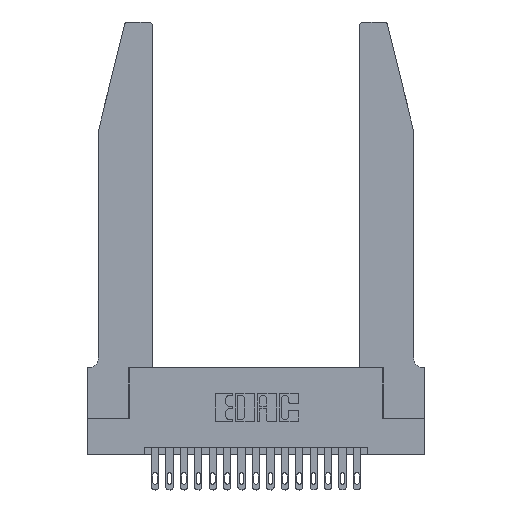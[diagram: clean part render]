
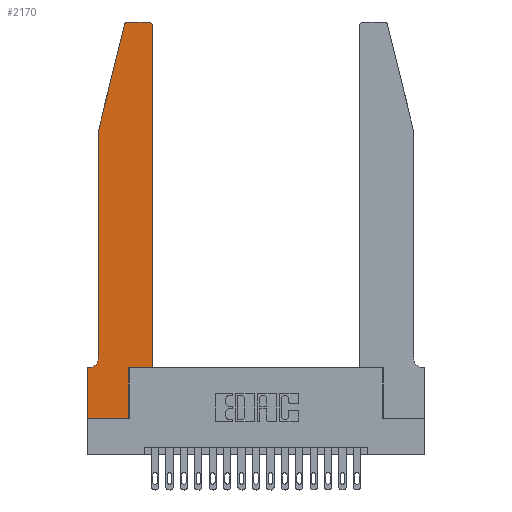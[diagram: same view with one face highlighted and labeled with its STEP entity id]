
A CAD part, top view. The second image highlights one B-rep face of the part: STEP entity #2170.
In plain terms, the highlighted planar face has unit normal (0, 0, 1).
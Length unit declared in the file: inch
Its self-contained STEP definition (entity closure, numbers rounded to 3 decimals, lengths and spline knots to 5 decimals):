
#248 = EDGE_CURVE ( 'NONE', #19533, #18526, #6119, .T. ) ;
#366 = DIRECTION ( 'NONE',  ( 1., 0., 0. ) ) ;
#376 = VERTEX_POINT ( 'NONE', #8955 ) ;
#439 = CARTESIAN_POINT ( 'NONE',  ( 0.0755, 0.35, 0.37 ) ) ;
#495 = VERTEX_POINT ( 'NONE', #17113 ) ;
#502 = EDGE_CURVE ( 'NONE', #8190, #19533, #6596, .T. ) ;
#740 = CARTESIAN_POINT ( 'NONE',  ( 0.2865, 0.35, 0.37 ) ) ;
#761 = ORIENTED_EDGE ( 'NONE', *, *, #19581, .T. ) ;
#892 = DIRECTION ( 'NONE',  ( -1., 0., 0. ) ) ;
#1048 = ORIENTED_EDGE ( 'NONE', *, *, #15730, .T. ) ;
#1582 = CARTESIAN_POINT ( 'NONE',  ( 0.0755, 0.42, 0.37 ) ) ;
#1654 = DIRECTION ( 'NONE',  ( 0., -1., 0. ) ) ;
#1697 = CARTESIAN_POINT ( 'NONE',  ( 0.4505, 0.35, 0.37 ) ) ;
#2170 = ADVANCED_FACE ( 'NONE', ( #5588 ), #3461, .T. ) ;
#3083 = EDGE_CURVE ( 'NONE', #18575, #8630, #14760, .T. ) ;
#3408 = AXIS2_PLACEMENT_3D ( 'NONE', #4958, #6515, #366 ) ;
#3455 = CARTESIAN_POINT ( 'NONE',  ( 0.4205, 2.75, 0.37 ) ) ;
#3461 = PLANE ( 'NONE',  #3408 ) ;
#3568 = CIRCLE ( 'NONE', #14250, 0.03 ) ;
#3593 = VERTEX_POINT ( 'NONE', #8522 ) ;
#3665 = LINE ( 'NONE', #19968, #15563 ) ;
#3952 = DIRECTION ( 'NONE',  ( 0., 0., 1. ) ) ;
#3953 = EDGE_CURVE ( 'NONE', #9859, #495, #4780, .T. ) ;
#4123 = EDGE_CURVE ( 'NONE', #14168, #9859, #5027, .T. ) ;
#4678 = CARTESIAN_POINT ( 'NONE',  ( 0., 0., 0.37 ) ) ;
#4702 = ORIENTED_EDGE ( 'NONE', *, *, #15828, .T. ) ;
#4780 = CIRCLE ( 'NONE', #11219, 0.07 ) ;
#4878 = CARTESIAN_POINT ( 'NONE',  ( 0.0755, 2., 0.37 ) ) ;
#4958 = CARTESIAN_POINT ( 'NONE',  ( 0., 0.35, 0.37 ) ) ;
#5027 = LINE ( 'NONE', #18552, #18361 ) ;
#5333 = EDGE_CURVE ( 'NONE', #3593, #18575, #12980, .T. ) ;
#5356 = ORIENTED_EDGE ( 'NONE', *, *, #248, .T. ) ;
#5588 = FACE_OUTER_BOUND ( 'NONE', #6091, .T. ) ;
#5661 = ORIENTED_EDGE ( 'NONE', *, *, #502, .T. ) ;
#5829 = LINE ( 'NONE', #8530, #14571 ) ;
#6091 = EDGE_LOOP ( 'NONE', ( #9227, #16138, #1048, #8426, #10344, #761, #7864, #5661, #5356, #4702, #13267, #17937 ) ) ;
#6119 = LINE ( 'NONE', #8564, #18029 ) ;
#6168 = VERTEX_POINT ( 'NONE', #17210 ) ;
#6281 = CARTESIAN_POINT ( 'NONE',  ( 0., 0., 0.37 ) ) ;
#6424 = DIRECTION ( 'NONE',  ( 0., 0., 1. ) ) ;
#6515 = DIRECTION ( 'NONE',  ( 0., 0., 1. ) ) ;
#6596 = LINE ( 'NONE', #17051, #9740 ) ;
#6760 = DIRECTION ( 'NONE',  ( 0., 0., -1. ) ) ;
#7532 = VECTOR ( 'NONE', #7723, 39.37008 ) ;
#7723 = DIRECTION ( 'NONE',  ( 1., 0., 0. ) ) ;
#7864 = ORIENTED_EDGE ( 'NONE', *, *, #14664, .T. ) ;
#8190 = VERTEX_POINT ( 'NONE', #4678 ) ;
#8325 = DIRECTION ( 'NONE',  ( -1., 0., 0. ) ) ;
#8426 = ORIENTED_EDGE ( 'NONE', *, *, #4123, .T. ) ;
#8522 = CARTESIAN_POINT ( 'NONE',  ( 0.4505, 0.35, 0.37 ) ) ;
#8530 = CARTESIAN_POINT ( 'NONE',  ( 0.2605, 2.75, 0.37 ) ) ;
#8564 = CARTESIAN_POINT ( 'NONE',  ( 0.2865, 0.35, 0.37 ) ) ;
#8630 = VERTEX_POINT ( 'NONE', #3455 ) ;
#8710 = DIRECTION ( 'NONE',  ( -1., 0., 0. ) ) ;
#8943 = DIRECTION ( 'NONE',  ( -0.239, -0.971, 0. ) ) ;
#8955 = CARTESIAN_POINT ( 'NONE',  ( 0.284, 2.75, 0.37 ) ) ;
#9227 = ORIENTED_EDGE ( 'NONE', *, *, #16183, .T. ) ;
#9392 = CARTESIAN_POINT ( 'NONE',  ( 0.4505, 0.35, 0.37 ) ) ;
#9740 = VECTOR ( 'NONE', #18667, 39.37008 ) ;
#9859 = VERTEX_POINT ( 'NONE', #1582 ) ;
#10344 = ORIENTED_EDGE ( 'NONE', *, *, #3953, .T. ) ;
#10961 = DIRECTION ( 'NONE',  ( 0., 1., 0. ) ) ;
#11219 = AXIS2_PLACEMENT_3D ( 'NONE', #14438, #6760, #8325 ) ;
#11280 = VECTOR ( 'NONE', #10961, 39.37008 ) ;
#11695 = CARTESIAN_POINT ( 'NONE',  ( 0.4505, 2.72, 0.37 ) ) ;
#11909 = LINE ( 'NONE', #6281, #18731 ) ;
#12718 = LINE ( 'NONE', #439, #13212 ) ;
#12980 = LINE ( 'NONE', #9392, #11280 ) ;
#13212 = VECTOR ( 'NONE', #8710, 39.37008 ) ;
#13255 = DIRECTION ( 'NONE',  ( 1., 0., 0. ) ) ;
#13267 = ORIENTED_EDGE ( 'NONE', *, *, #5333, .T. ) ;
#13308 = AXIS2_PLACEMENT_3D ( 'NONE', #16372, #3952, #13255 ) ;
#14168 = VERTEX_POINT ( 'NONE', #4878 ) ;
#14250 = AXIS2_PLACEMENT_3D ( 'NONE', #18914, #6424, #14300 ) ;
#14300 = DIRECTION ( 'NONE',  ( 1., 0., 0. ) ) ;
#14438 = CARTESIAN_POINT ( 'NONE',  ( 0.0055, 0.42, 0.37 ) ) ;
#14571 = VECTOR ( 'NONE', #892, 39.37008 ) ;
#14664 = EDGE_CURVE ( 'NONE', #6168, #8190, #11909, .T. ) ;
#14737 = DIRECTION ( 'NONE',  ( 0., 1., 0. ) ) ;
#14760 = CIRCLE ( 'NONE', #13308, 0.03 ) ;
#15054 = LINE ( 'NONE', #1697, #7532 ) ;
#15381 = DIRECTION ( 'NONE',  ( 0., -1., 0. ) ) ;
#15563 = VECTOR ( 'NONE', #8943, 39.37008 ) ;
#15730 = EDGE_CURVE ( 'NONE', #16727, #14168, #3665, .T. ) ;
#15828 = EDGE_CURVE ( 'NONE', #18526, #3593, #15054, .T. ) ;
#16138 = ORIENTED_EDGE ( 'NONE', *, *, #18351, .T. ) ;
#16183 = EDGE_CURVE ( 'NONE', #8630, #376, #5829, .T. ) ;
#16372 = CARTESIAN_POINT ( 'NONE',  ( 0.4205, 2.72, 0.37 ) ) ;
#16727 = VERTEX_POINT ( 'NONE', #17481 ) ;
#17051 = CARTESIAN_POINT ( 'NONE',  ( 0., 0., 0.37 ) ) ;
#17113 = CARTESIAN_POINT ( 'NONE',  ( 0.0055, 0.35, 0.37 ) ) ;
#17210 = CARTESIAN_POINT ( 'NONE',  ( 0., 0.35, 0.37 ) ) ;
#17481 = CARTESIAN_POINT ( 'NONE',  ( 0.25487, 2.72718, 0.37 ) ) ;
#17937 = ORIENTED_EDGE ( 'NONE', *, *, #3083, .T. ) ;
#18029 = VECTOR ( 'NONE', #14737, 39.37008 ) ;
#18351 = EDGE_CURVE ( 'NONE', #376, #16727, #3568, .T. ) ;
#18361 = VECTOR ( 'NONE', #1654, 39.37008 ) ;
#18526 = VERTEX_POINT ( 'NONE', #740 ) ;
#18552 = CARTESIAN_POINT ( 'NONE',  ( 0.0755, 2., 0.37 ) ) ;
#18575 = VERTEX_POINT ( 'NONE', #11695 ) ;
#18667 = DIRECTION ( 'NONE',  ( 1., 0., 0. ) ) ;
#18731 = VECTOR ( 'NONE', #15381, 39.37008 ) ;
#18842 = CARTESIAN_POINT ( 'NONE',  ( 0.2865, 0., 0.37 ) ) ;
#18914 = CARTESIAN_POINT ( 'NONE',  ( 0.284, 2.72, 0.37 ) ) ;
#19533 = VERTEX_POINT ( 'NONE', #18842 ) ;
#19581 = EDGE_CURVE ( 'NONE', #495, #6168, #12718, .T. ) ;
#19968 = CARTESIAN_POINT ( 'NONE',  ( 0.0755, 2., 0.37 ) ) ;
